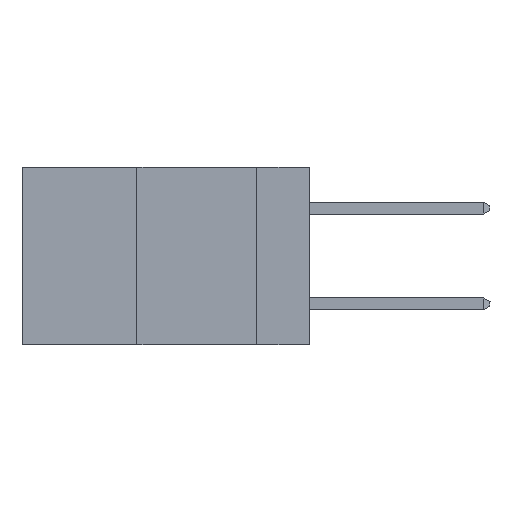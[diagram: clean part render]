
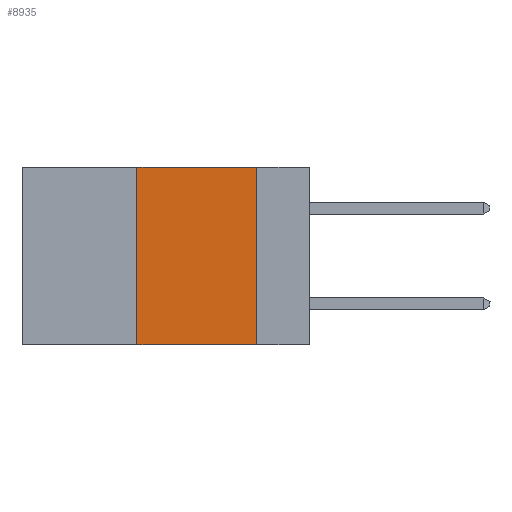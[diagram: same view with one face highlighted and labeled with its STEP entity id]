
A CAD part, left-side view. The second image highlights one B-rep face of the part: STEP entity #8935.
In plain terms, the highlighted planar face has unit normal (-1, 0, 0).
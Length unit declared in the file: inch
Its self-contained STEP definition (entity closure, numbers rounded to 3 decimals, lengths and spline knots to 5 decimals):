
#419 = PLANE ( 'NONE',  #13083 ) ;
#648 = DIRECTION ( 'NONE',  ( 0., 0., -1. ) ) ;
#977 = VERTEX_POINT ( 'NONE', #4638 ) ;
#1653 = CARTESIAN_POINT ( 'NONE',  ( 0., 0.36, 0. ) ) ;
#4638 = CARTESIAN_POINT ( 'NONE',  ( 0., 0.11, -0.37 ) ) ;
#6661 = EDGE_CURVE ( 'NONE', #24661, #977, #39012, .T. ) ;
#6781 = LINE ( 'NONE', #31943, #29335 ) ;
#7293 = CARTESIAN_POINT ( 'NONE',  ( 0., 0.36, 0. ) ) ;
#8935 = ADVANCED_FACE ( 'NONE', ( #25381 ), #419, .F. ) ;
#8997 = DIRECTION ( 'NONE',  ( 0., 0., 1. ) ) ;
#9210 = LINE ( 'NONE', #1653, #25787 ) ;
#9230 = VECTOR ( 'NONE', #45189, 39.37008 ) ;
#9795 = DIRECTION ( 'NONE',  ( 0., -1., 0. ) ) ;
#10166 = ORIENTED_EDGE ( 'NONE', *, *, #22423, .F. ) ;
#10804 = ORIENTED_EDGE ( 'NONE', *, *, #6661, .T. ) ;
#13083 = AXIS2_PLACEMENT_3D ( 'NONE', #21952, #36169, #648 ) ;
#19260 = ORIENTED_EDGE ( 'NONE', *, *, #33073, .F. ) ;
#19778 = VECTOR ( 'NONE', #9795, 39.37008 ) ;
#21952 = CARTESIAN_POINT ( 'NONE',  ( 0., 0.6, 0. ) ) ;
#22406 = CARTESIAN_POINT ( 'NONE',  ( 0., 0.36, -0.37 ) ) ;
#22423 = EDGE_CURVE ( 'NONE', #24661, #38114, #9210, .T. ) ;
#24557 = CARTESIAN_POINT ( 'NONE',  ( 0., 0.6, -0.37 ) ) ;
#24661 = VERTEX_POINT ( 'NONE', #22406 ) ;
#25381 = FACE_OUTER_BOUND ( 'NONE', #35548, .T. ) ;
#25787 = VECTOR ( 'NONE', #8997, 39.37008 ) ;
#26366 = CARTESIAN_POINT ( 'NONE',  ( 0., 0.11, 0. ) ) ;
#29335 = VECTOR ( 'NONE', #38388, 39.37008 ) ;
#31943 = CARTESIAN_POINT ( 'NONE',  ( 0., 0.11, 0. ) ) ;
#33073 = EDGE_CURVE ( 'NONE', #38114, #34030, #44846, .T. ) ;
#33895 = EDGE_CURVE ( 'NONE', #34030, #977, #6781, .T. ) ;
#34030 = VERTEX_POINT ( 'NONE', #26366 ) ;
#34527 = CARTESIAN_POINT ( 'NONE',  ( 0., 0.6, 0. ) ) ;
#35548 = EDGE_LOOP ( 'NONE', ( #40639, #19260, #10166, #10804 ) ) ;
#36169 = DIRECTION ( 'NONE',  ( 1., 0., 0. ) ) ;
#38114 = VERTEX_POINT ( 'NONE', #7293 ) ;
#38388 = DIRECTION ( 'NONE',  ( 0., 0., -1. ) ) ;
#39012 = LINE ( 'NONE', #24557, #9230 ) ;
#40639 = ORIENTED_EDGE ( 'NONE', *, *, #33895, .F. ) ;
#44846 = LINE ( 'NONE', #34527, #19778 ) ;
#45189 = DIRECTION ( 'NONE',  ( 0., -1., 0. ) ) ;
